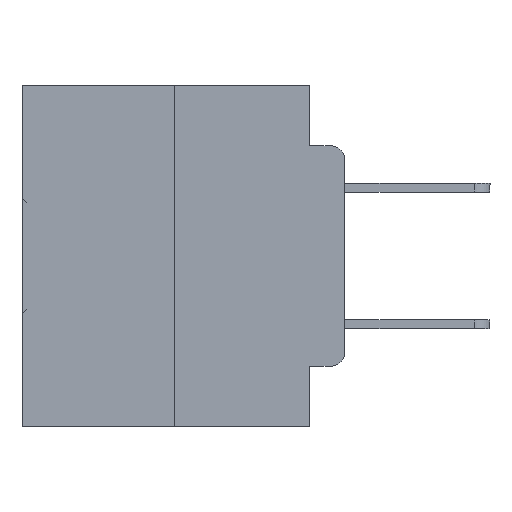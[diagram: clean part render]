
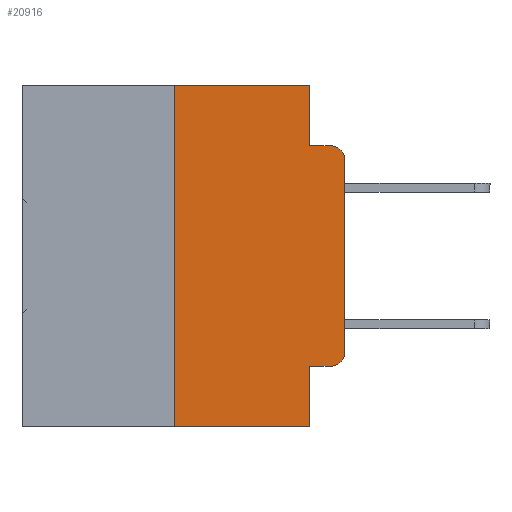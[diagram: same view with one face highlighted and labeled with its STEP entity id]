
A CAD part, left-side view. The second image highlights one B-rep face of the part: STEP entity #20916.
In plain terms, the highlighted planar face has unit normal (-1, 0, 0).
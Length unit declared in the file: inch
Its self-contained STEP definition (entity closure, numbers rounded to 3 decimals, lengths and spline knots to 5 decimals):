
#274 = AXIS2_PLACEMENT_3D ( 'NONE', #2908, #20393, #5453 ) ;
#1869 = CARTESIAN_POINT ( 'NONE',  ( 0., 0.25, 0. ) ) ;
#2448 = VERTEX_POINT ( 'NONE', #28013 ) ;
#2626 = DIRECTION ( 'NONE',  ( 0., 0., -1. ) ) ;
#2664 = VECTOR ( 'NONE', #16809, 39.37008 ) ;
#2704 = CARTESIAN_POINT ( 'NONE',  ( 0., 0., -0.1085 ) ) ;
#2883 = EDGE_CURVE ( 'NONE', #17080, #22644, #16035, .T. ) ;
#2908 = CARTESIAN_POINT ( 'NONE',  ( 0., 0.02, -0.3915 ) ) ;
#3016 = FACE_OUTER_BOUND ( 'NONE', #22412, .T. ) ;
#3516 = VERTEX_POINT ( 'NONE', #4471 ) ;
#3677 = VECTOR ( 'NONE', #2626, 39.37008 ) ;
#4320 = VERTEX_POINT ( 'NONE', #13335 ) ;
#4352 = VERTEX_POINT ( 'NONE', #29480 ) ;
#4471 = CARTESIAN_POINT ( 'NONE',  ( 0., 0.02, -0.4115 ) ) ;
#4842 = VECTOR ( 'NONE', #19072, 39.37008 ) ;
#5143 = ORIENTED_EDGE ( 'NONE', *, *, #8376, .T. ) ;
#5453 = DIRECTION ( 'NONE',  ( 0., 0., -1. ) ) ;
#5555 = ORIENTED_EDGE ( 'NONE', *, *, #31814, .T. ) ;
#5645 = LINE ( 'NONE', #21554, #4842 ) ;
#5945 = AXIS2_PLACEMENT_3D ( 'NONE', #18674, #11251, #28630 ) ;
#6592 = CARTESIAN_POINT ( 'NONE',  ( 0., 0., -0.3915 ) ) ;
#6958 = DIRECTION ( 'NONE',  ( 0., 0., 1. ) ) ;
#7522 = VERTEX_POINT ( 'NONE', #12177 ) ;
#8253 = VERTEX_POINT ( 'NONE', #14350 ) ;
#8286 = CARTESIAN_POINT ( 'NONE',  ( 0., 0.051, 0. ) ) ;
#8289 = ORIENTED_EDGE ( 'NONE', *, *, #28563, .F. ) ;
#8376 = EDGE_CURVE ( 'NONE', #2448, #16952, #17932, .T. ) ;
#9270 = CARTESIAN_POINT ( 'NONE',  ( 0., 0.02, -0.1085 ) ) ;
#9303 = CARTESIAN_POINT ( 'NONE',  ( 0., 0., 0. ) ) ;
#10353 = AXIS2_PLACEMENT_3D ( 'NONE', #9270, #26638, #11775 ) ;
#10643 = ORIENTED_EDGE ( 'NONE', *, *, #30200, .F. ) ;
#10985 = CIRCLE ( 'NONE', #274, 0.02 ) ;
#11251 = DIRECTION ( 'NONE',  ( 1., 0., 0. ) ) ;
#11291 = VECTOR ( 'NONE', #18922, 39.37008 ) ;
#11775 = DIRECTION ( 'NONE',  ( 0., 0., -1. ) ) ;
#12177 = CARTESIAN_POINT ( 'NONE',  ( 0., 0.051, 0. ) ) ;
#13335 = CARTESIAN_POINT ( 'NONE',  ( 0., 0.25, 0. ) ) ;
#13401 = LINE ( 'NONE', #1869, #20002 ) ;
#14350 = CARTESIAN_POINT ( 'NONE',  ( 0., 0.02, -0.0885 ) ) ;
#15238 = ORIENTED_EDGE ( 'NONE', *, *, #18609, .T. ) ;
#15971 = CIRCLE ( 'NONE', #10353, 0.02 ) ;
#16035 = LINE ( 'NONE', #9303, #17599 ) ;
#16412 = CARTESIAN_POINT ( 'NONE',  ( 0., 0.473, -0.5 ) ) ;
#16540 = EDGE_CURVE ( 'NONE', #4320, #7522, #5645, .T. ) ;
#16809 = DIRECTION ( 'NONE',  ( 0., -1., 0. ) ) ;
#16895 = LINE ( 'NONE', #17324, #25072 ) ;
#16952 = VERTEX_POINT ( 'NONE', #25982 ) ;
#17080 = VERTEX_POINT ( 'NONE', #6592 ) ;
#17234 = ORIENTED_EDGE ( 'NONE', *, *, #21917, .F. ) ;
#17324 = CARTESIAN_POINT ( 'NONE',  ( 0., 0.051, -0.0885 ) ) ;
#17599 = VECTOR ( 'NONE', #26670, 39.37008 ) ;
#17635 = CARTESIAN_POINT ( 'NONE',  ( 0., 0.051, 0. ) ) ;
#17932 = LINE ( 'NONE', #16412, #11291 ) ;
#17934 = ORIENTED_EDGE ( 'NONE', *, *, #20265, .T. ) ;
#18609 = EDGE_CURVE ( 'NONE', #3516, #17080, #10985, .T. ) ;
#18674 = CARTESIAN_POINT ( 'NONE',  ( 0., 0.473, 0. ) ) ;
#18922 = DIRECTION ( 'NONE',  ( 0., -1., 0. ) ) ;
#19072 = DIRECTION ( 'NONE',  ( 0., -1., 0. ) ) ;
#19200 = ORIENTED_EDGE ( 'NONE', *, *, #23598, .F. ) ;
#20002 = VECTOR ( 'NONE', #6958, 39.37008 ) ;
#20265 = EDGE_CURVE ( 'NONE', #26828, #3516, #21813, .T. ) ;
#20393 = DIRECTION ( 'NONE',  ( -1., 0., 0. ) ) ;
#20700 = DIRECTION ( 'NONE',  ( 0., 0., -1. ) ) ;
#20916 = ADVANCED_FACE ( 'NONE', ( #3016 ), #21159, .F. ) ;
#21159 = PLANE ( 'NONE',  #5945 ) ;
#21554 = CARTESIAN_POINT ( 'NONE',  ( 0., 0.473, 0. ) ) ;
#21813 = LINE ( 'NONE', #24325, #2664 ) ;
#21917 = EDGE_CURVE ( 'NONE', #26828, #16952, #23617, .T. ) ;
#22412 = EDGE_LOOP ( 'NONE', ( #27748, #5555, #10643, #8289, #27343, #19200, #5143, #17234, #17934, #15238 ) ) ;
#22644 = VERTEX_POINT ( 'NONE', #2704 ) ;
#23598 = EDGE_CURVE ( 'NONE', #2448, #4320, #13401, .T. ) ;
#23617 = LINE ( 'NONE', #17635, #3677 ) ;
#24325 = CARTESIAN_POINT ( 'NONE',  ( 0., 0.051, -0.4115 ) ) ;
#25072 = VECTOR ( 'NONE', #27293, 39.37008 ) ;
#25550 = VECTOR ( 'NONE', #20700, 39.37008 ) ;
#25982 = CARTESIAN_POINT ( 'NONE',  ( 0., 0.051, -0.5 ) ) ;
#26300 = LINE ( 'NONE', #8286, #25550 ) ;
#26638 = DIRECTION ( 'NONE',  ( -1., 0., 0. ) ) ;
#26670 = DIRECTION ( 'NONE',  ( 0., 0., 1. ) ) ;
#26828 = VERTEX_POINT ( 'NONE', #31355 ) ;
#27293 = DIRECTION ( 'NONE',  ( 0., -1., 0. ) ) ;
#27343 = ORIENTED_EDGE ( 'NONE', *, *, #16540, .F. ) ;
#27748 = ORIENTED_EDGE ( 'NONE', *, *, #2883, .T. ) ;
#28013 = CARTESIAN_POINT ( 'NONE',  ( 0., 0.25, -0.5 ) ) ;
#28563 = EDGE_CURVE ( 'NONE', #7522, #4352, #26300, .T. ) ;
#28630 = DIRECTION ( 'NONE',  ( 0., 0., -1. ) ) ;
#29480 = CARTESIAN_POINT ( 'NONE',  ( 0., 0.051, -0.0885 ) ) ;
#30200 = EDGE_CURVE ( 'NONE', #4352, #8253, #16895, .T. ) ;
#31355 = CARTESIAN_POINT ( 'NONE',  ( 0., 0.051, -0.4115 ) ) ;
#31814 = EDGE_CURVE ( 'NONE', #22644, #8253, #15971, .T. ) ;
